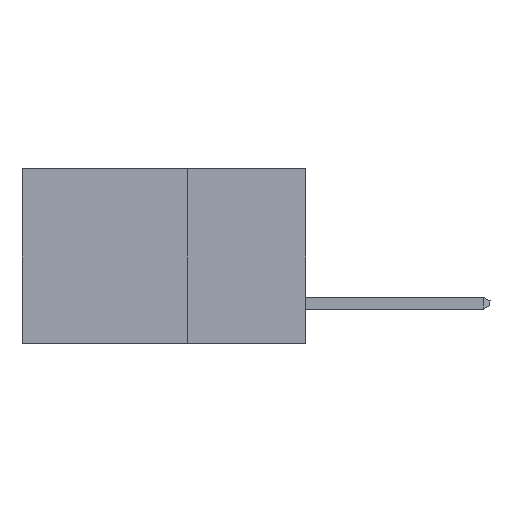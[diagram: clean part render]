
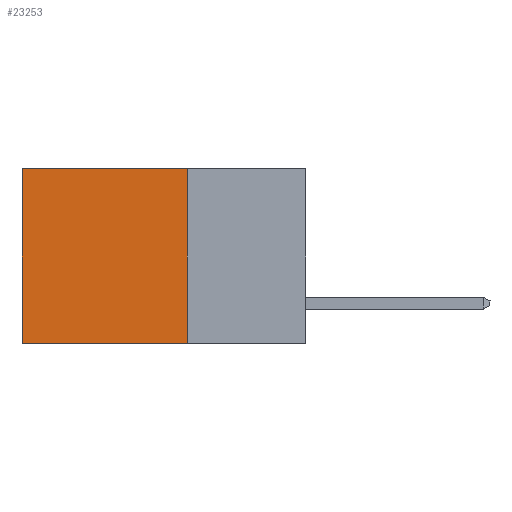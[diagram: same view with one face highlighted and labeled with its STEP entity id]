
A CAD part, left-side view. The second image highlights one B-rep face of the part: STEP entity #23253.
In plain terms, the highlighted planar face has unit normal (-1, 0, 0).
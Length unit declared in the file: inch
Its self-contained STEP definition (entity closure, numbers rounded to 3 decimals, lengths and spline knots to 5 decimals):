
#644 = DIRECTION ( 'NONE',  ( 0., 0., -1. ) ) ;
#1572 = DIRECTION ( 'NONE',  ( 0., 1., 0. ) ) ;
#2583 = VECTOR ( 'NONE', #4442, 39.37008 ) ;
#3519 = ORIENTED_EDGE ( 'NONE', *, *, #10513, .F. ) ;
#3707 = EDGE_CURVE ( 'NONE', #17956, #4938, #16586, .T. ) ;
#3936 = CARTESIAN_POINT ( 'NONE',  ( 0.2615, 0.6, -0.37 ) ) ;
#3996 = VERTEX_POINT ( 'NONE', #19998 ) ;
#4442 = DIRECTION ( 'NONE',  ( 0., 1., 0. ) ) ;
#4843 = EDGE_CURVE ( 'NONE', #3996, #4938, #10611, .T. ) ;
#4938 = VERTEX_POINT ( 'NONE', #3936 ) ;
#5131 = ORIENTED_EDGE ( 'NONE', *, *, #7142, .T. ) ;
#5339 = LINE ( 'NONE', #20033, #10475 ) ;
#5803 = CARTESIAN_POINT ( 'NONE',  ( 0.2615, 0.25, 0. ) ) ;
#7142 = EDGE_CURVE ( 'NONE', #13199, #3996, #7797, .T. ) ;
#7797 = LINE ( 'NONE', #5803, #2583 ) ;
#7824 = CARTESIAN_POINT ( 'NONE',  ( 0.2615, 0.25, -0.37 ) ) ;
#10267 = CARTESIAN_POINT ( 'NONE',  ( 0.2615, 0.6, -0.37 ) ) ;
#10475 = VECTOR ( 'NONE', #19999, 39.37008 ) ;
#10513 = EDGE_CURVE ( 'NONE', #13199, #17956, #5339, .T. ) ;
#10611 = LINE ( 'NONE', #10267, #20978 ) ;
#11300 = VECTOR ( 'NONE', #1572, 39.37008 ) ;
#12227 = ORIENTED_EDGE ( 'NONE', *, *, #3707, .F. ) ;
#12252 = CARTESIAN_POINT ( 'NONE',  ( 0.2615, 0.25, -0.37 ) ) ;
#12327 = DIRECTION ( 'NONE',  ( 1., 0., 0. ) ) ;
#12589 = ORIENTED_EDGE ( 'NONE', *, *, #4843, .T. ) ;
#13192 = EDGE_LOOP ( 'NONE', ( #12589, #12227, #3519, #5131 ) ) ;
#13199 = VERTEX_POINT ( 'NONE', #22615 ) ;
#13815 = DIRECTION ( 'NONE',  ( 0., 0., -1. ) ) ;
#14954 = FACE_OUTER_BOUND ( 'NONE', #13192, .T. ) ;
#16586 = LINE ( 'NONE', #22168, #11300 ) ;
#17956 = VERTEX_POINT ( 'NONE', #7824 ) ;
#19998 = CARTESIAN_POINT ( 'NONE',  ( 0.2615, 0.6, 0. ) ) ;
#19999 = DIRECTION ( 'NONE',  ( 0., 0., -1. ) ) ;
#20033 = CARTESIAN_POINT ( 'NONE',  ( 0.2615, 0.25, -0.37 ) ) ;
#20096 = PLANE ( 'NONE',  #21230 ) ;
#20978 = VECTOR ( 'NONE', #13815, 39.37008 ) ;
#21230 = AXIS2_PLACEMENT_3D ( 'NONE', #12252, #12327, #644 ) ;
#22168 = CARTESIAN_POINT ( 'NONE',  ( 0.2615, 0.25, -0.37 ) ) ;
#22615 = CARTESIAN_POINT ( 'NONE',  ( 0.2615, 0.25, 0. ) ) ;
#23253 = ADVANCED_FACE ( 'NONE', ( #14954 ), #20096, .F. ) ;
